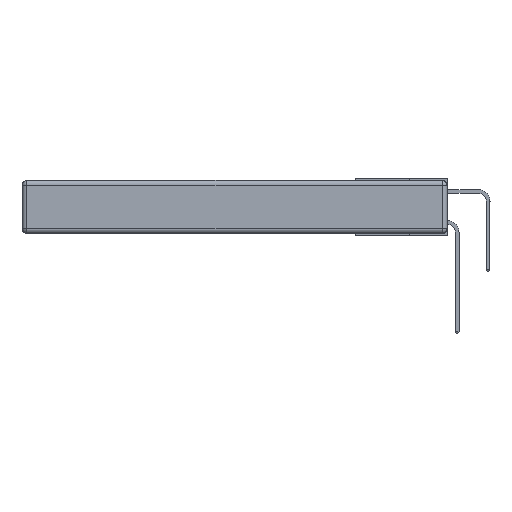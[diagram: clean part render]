
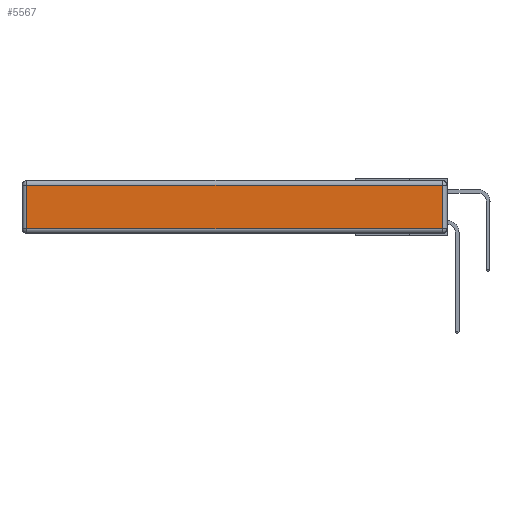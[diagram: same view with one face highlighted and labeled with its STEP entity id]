
A CAD part, left-side view. The second image highlights one B-rep face of the part: STEP entity #5567.
In plain terms, the highlighted planar face has unit normal (-1, 0, 0).
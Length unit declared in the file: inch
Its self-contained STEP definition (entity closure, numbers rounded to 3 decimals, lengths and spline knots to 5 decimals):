
#1248 = VECTOR ( 'NONE', #5152, 39.37008 ) ;
#1362 = ORIENTED_EDGE ( 'NONE', *, *, #15903, .T. ) ;
#1506 = CARTESIAN_POINT ( 'NONE',  ( 0., 2.72, -0.03 ) ) ;
#1533 = ORIENTED_EDGE ( 'NONE', *, *, #19180, .T. ) ;
#1908 = DIRECTION ( 'NONE',  ( 0., 0., 1. ) ) ;
#2442 = CARTESIAN_POINT ( 'NONE',  ( 0., 0.03, -0.03 ) ) ;
#2696 = LINE ( 'NONE', #19188, #9360 ) ;
#5152 = DIRECTION ( 'NONE',  ( 0., 1., 0. ) ) ;
#5567 = ADVANCED_FACE ( 'NONE', ( #11572 ), #23887, .T. ) ;
#5601 = DIRECTION ( 'NONE',  ( 0., 0., 1. ) ) ;
#5895 = CARTESIAN_POINT ( 'NONE',  ( 0., 0.03, -0.343 ) ) ;
#6367 = VERTEX_POINT ( 'NONE', #23961 ) ;
#7346 = VECTOR ( 'NONE', #12697, 39.37008 ) ;
#7537 = AXIS2_PLACEMENT_3D ( 'NONE', #15771, #20108, #5601 ) ;
#7906 = LINE ( 'NONE', #5895, #23388 ) ;
#8452 = VERTEX_POINT ( 'NONE', #1506 ) ;
#9360 = VECTOR ( 'NONE', #23258, 39.37008 ) ;
#11006 = ORIENTED_EDGE ( 'NONE', *, *, #24057, .T. ) ;
#11572 = FACE_OUTER_BOUND ( 'NONE', #14492, .T. ) ;
#12697 = DIRECTION ( 'NONE',  ( 0., -1., 0. ) ) ;
#12795 = VERTEX_POINT ( 'NONE', #24135 ) ;
#14142 = ORIENTED_EDGE ( 'NONE', *, *, #23122, .T. ) ;
#14333 = LINE ( 'NONE', #14646, #7346 ) ;
#14492 = EDGE_LOOP ( 'NONE', ( #14142, #1533, #11006, #1362 ) ) ;
#14646 = CARTESIAN_POINT ( 'NONE',  ( 0., 0., -0.313 ) ) ;
#15520 = VERTEX_POINT ( 'NONE', #2442 ) ;
#15771 = CARTESIAN_POINT ( 'NONE',  ( 0., 0., -0.343 ) ) ;
#15903 = EDGE_CURVE ( 'NONE', #8452, #12795, #2696, .T. ) ;
#19180 = EDGE_CURVE ( 'NONE', #6367, #15520, #7906, .T. ) ;
#19188 = CARTESIAN_POINT ( 'NONE',  ( 0., 2.72, -0.343 ) ) ;
#20108 = DIRECTION ( 'NONE',  ( -1., 0., 0. ) ) ;
#20572 = LINE ( 'NONE', #25188, #1248 ) ;
#23122 = EDGE_CURVE ( 'NONE', #12795, #6367, #14333, .T. ) ;
#23258 = DIRECTION ( 'NONE',  ( 0., 0., -1. ) ) ;
#23388 = VECTOR ( 'NONE', #1908, 39.37008 ) ;
#23887 = PLANE ( 'NONE',  #7537 ) ;
#23961 = CARTESIAN_POINT ( 'NONE',  ( 0., 0.03, -0.313 ) ) ;
#24057 = EDGE_CURVE ( 'NONE', #15520, #8452, #20572, .T. ) ;
#24135 = CARTESIAN_POINT ( 'NONE',  ( 0., 2.72, -0.313 ) ) ;
#25188 = CARTESIAN_POINT ( 'NONE',  ( 0., 2.75, -0.03 ) ) ;
